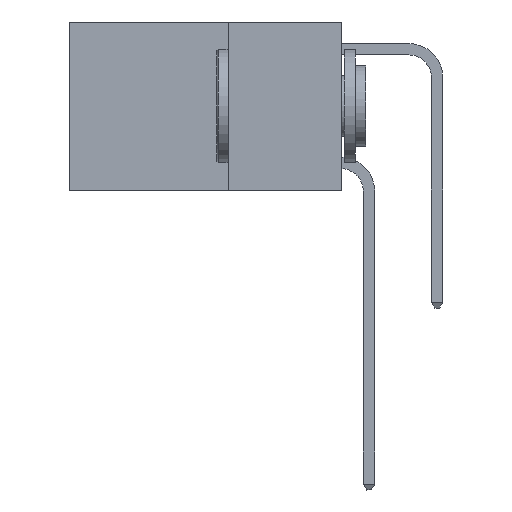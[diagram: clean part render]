
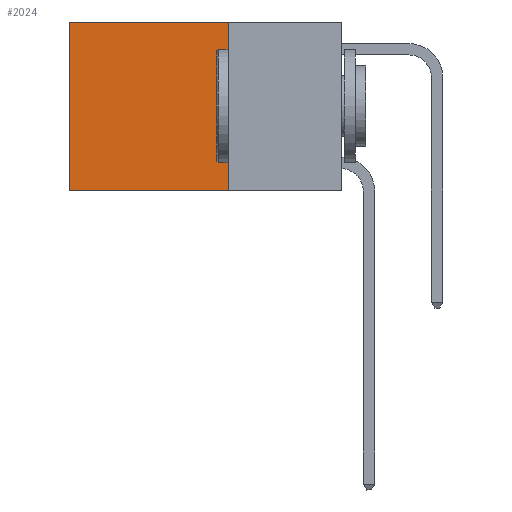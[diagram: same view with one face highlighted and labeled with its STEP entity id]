
A CAD part, left-side view. The second image highlights one B-rep face of the part: STEP entity #2024.
In plain terms, the highlighted planar face has unit normal (-1, 0, 0).
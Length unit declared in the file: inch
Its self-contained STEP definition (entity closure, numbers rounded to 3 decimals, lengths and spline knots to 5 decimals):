
#12 = CARTESIAN_POINT ( 'NONE',  ( 0.2625, 0.25, 0. ) ) ;
#80 = CARTESIAN_POINT ( 'NONE',  ( 0.2625, 0.25, 0. ) ) ;
#226 = CARTESIAN_POINT ( 'NONE',  ( 0.2625, 0.25, 0. ) ) ;
#863 = VERTEX_POINT ( 'NONE', #5859 ) ;
#1310 = CARTESIAN_POINT ( 'NONE',  ( 0.2625, 0.25, -0.37 ) ) ;
#1503 = ORIENTED_EDGE ( 'NONE', *, *, #20281, .F. ) ;
#2024 = ADVANCED_FACE ( 'NONE', ( #11998 ), #23522, .F. ) ;
#2439 = ORIENTED_EDGE ( 'NONE', *, *, #11553, .T. ) ;
#2744 = VECTOR ( 'NONE', #23274, 39.37008 ) ;
#3173 = DIRECTION ( 'NONE',  ( 0., 0., -1. ) ) ;
#5140 = VECTOR ( 'NONE', #3173, 39.37008 ) ;
#5840 = LINE ( 'NONE', #226, #20084 ) ;
#5859 = CARTESIAN_POINT ( 'NONE',  ( 0.2625, 0.6, 0. ) ) ;
#5975 = CARTESIAN_POINT ( 'NONE',  ( 0.2625, 0.6, 0. ) ) ;
#6517 = DIRECTION ( 'NONE',  ( 1., 0., 0. ) ) ;
#8631 = LINE ( 'NONE', #1310, #2744 ) ;
#8899 = ORIENTED_EDGE ( 'NONE', *, *, #17379, .F. ) ;
#9436 = DIRECTION ( 'NONE',  ( 0., 1., 0. ) ) ;
#11553 = EDGE_CURVE ( 'NONE', #16679, #863, #5840, .T. ) ;
#11998 = FACE_OUTER_BOUND ( 'NONE', #22613, .T. ) ;
#12618 = VECTOR ( 'NONE', #20751, 39.37008 ) ;
#13142 = CARTESIAN_POINT ( 'NONE',  ( 0.2625, 0.6, -0.37 ) ) ;
#13534 = ORIENTED_EDGE ( 'NONE', *, *, #16425, .T. ) ;
#16393 = DIRECTION ( 'NONE',  ( 0., 0., -1. ) ) ;
#16425 = EDGE_CURVE ( 'NONE', #863, #17601, #16961, .T. ) ;
#16679 = VERTEX_POINT ( 'NONE', #80 ) ;
#16961 = LINE ( 'NONE', #5975, #12618 ) ;
#17379 = EDGE_CURVE ( 'NONE', #23468, #17601, #8631, .T. ) ;
#17601 = VERTEX_POINT ( 'NONE', #13142 ) ;
#17736 = LINE ( 'NONE', #21315, #5140 ) ;
#18722 = AXIS2_PLACEMENT_3D ( 'NONE', #12, #6517, #16393 ) ;
#20084 = VECTOR ( 'NONE', #9436, 39.37008 ) ;
#20281 = EDGE_CURVE ( 'NONE', #16679, #23468, #17736, .T. ) ;
#20751 = DIRECTION ( 'NONE',  ( 0., 0., -1. ) ) ;
#21315 = CARTESIAN_POINT ( 'NONE',  ( 0.2625, 0.25, 0. ) ) ;
#22162 = CARTESIAN_POINT ( 'NONE',  ( 0.2625, 0.25, -0.37 ) ) ;
#22613 = EDGE_LOOP ( 'NONE', ( #13534, #8899, #1503, #2439 ) ) ;
#23274 = DIRECTION ( 'NONE',  ( 0., 1., 0. ) ) ;
#23468 = VERTEX_POINT ( 'NONE', #22162 ) ;
#23522 = PLANE ( 'NONE',  #18722 ) ;
